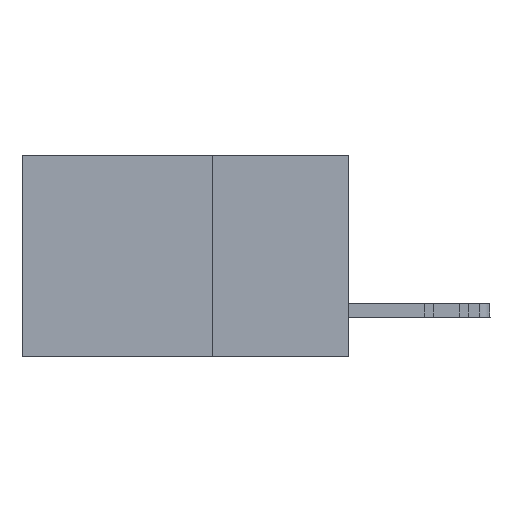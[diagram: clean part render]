
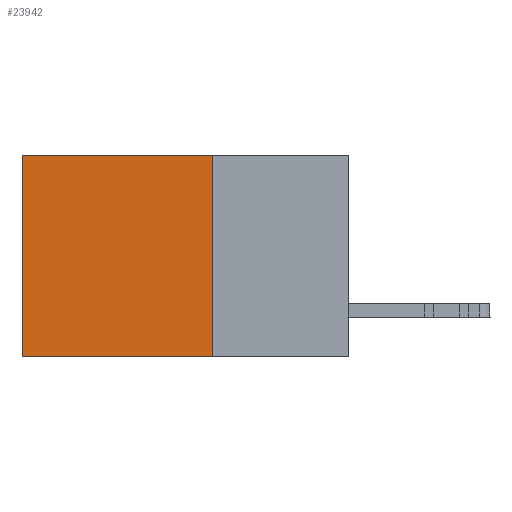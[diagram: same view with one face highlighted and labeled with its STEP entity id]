
A CAD part, left-side view. The second image highlights one B-rep face of the part: STEP entity #23942.
In plain terms, the highlighted planar face has unit normal (-1, 0, 0).
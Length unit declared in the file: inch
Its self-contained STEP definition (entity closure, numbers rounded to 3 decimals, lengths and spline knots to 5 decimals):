
#13 = DIRECTION ( 'NONE',  ( 1., 0., 0. ) ) ;
#1052 = EDGE_CURVE ( 'NONE', #3298, #9524, #8488, .T. ) ;
#1216 = VERTEX_POINT ( 'NONE', #14364 ) ;
#2584 = DIRECTION ( 'NONE',  ( 0., 0., -1. ) ) ;
#2949 = EDGE_CURVE ( 'NONE', #5682, #3298, #21023, .T. ) ;
#3145 = CARTESIAN_POINT ( 'NONE',  ( 0.298, 0.25, -0.37 ) ) ;
#3233 = VECTOR ( 'NONE', #11084, 39.37008 ) ;
#3298 = VERTEX_POINT ( 'NONE', #3145 ) ;
#4064 = DIRECTION ( 'NONE',  ( 0., 0., -1. ) ) ;
#4912 = FACE_OUTER_BOUND ( 'NONE', #11764, .T. ) ;
#4947 = VECTOR ( 'NONE', #11719, 39.37008 ) ;
#5124 = CARTESIAN_POINT ( 'NONE',  ( 0.298, 0.25, 0. ) ) ;
#5374 = CARTESIAN_POINT ( 'NONE',  ( 0.298, 0.6, -0.37 ) ) ;
#5555 = CARTESIAN_POINT ( 'NONE',  ( 0.298, 0.6, 0. ) ) ;
#5682 = VERTEX_POINT ( 'NONE', #8349 ) ;
#5852 = ORIENTED_EDGE ( 'NONE', *, *, #26407, .T. ) ;
#6251 = CARTESIAN_POINT ( 'NONE',  ( 0.298, 0.25, 0. ) ) ;
#6749 = VECTOR ( 'NONE', #2584, 39.37008 ) ;
#7131 = LINE ( 'NONE', #5124, #3233 ) ;
#7224 = EDGE_CURVE ( 'NONE', #5682, #1216, #7131, .T. ) ;
#8349 = CARTESIAN_POINT ( 'NONE',  ( 0.298, 0.25, 0. ) ) ;
#8488 = LINE ( 'NONE', #19992, #4947 ) ;
#8994 = LINE ( 'NONE', #5555, #22265 ) ;
#9524 = VERTEX_POINT ( 'NONE', #5374 ) ;
#9653 = ORIENTED_EDGE ( 'NONE', *, *, #1052, .F. ) ;
#11084 = DIRECTION ( 'NONE',  ( 0., 1., 0. ) ) ;
#11719 = DIRECTION ( 'NONE',  ( 0., 1., 0. ) ) ;
#11764 = EDGE_LOOP ( 'NONE', ( #5852, #9653, #14864, #23174 ) ) ;
#14364 = CARTESIAN_POINT ( 'NONE',  ( 0.298, 0.6, 0. ) ) ;
#14864 = ORIENTED_EDGE ( 'NONE', *, *, #2949, .F. ) ;
#19992 = CARTESIAN_POINT ( 'NONE',  ( 0.298, 0.25, -0.37 ) ) ;
#20626 = PLANE ( 'NONE',  #20905 ) ;
#20905 = AXIS2_PLACEMENT_3D ( 'NONE', #6251, #13, #4064 ) ;
#21023 = LINE ( 'NONE', #23589, #6749 ) ;
#22265 = VECTOR ( 'NONE', #24212, 39.37008 ) ;
#23174 = ORIENTED_EDGE ( 'NONE', *, *, #7224, .T. ) ;
#23589 = CARTESIAN_POINT ( 'NONE',  ( 0.298, 0.25, 0. ) ) ;
#23942 = ADVANCED_FACE ( 'NONE', ( #4912 ), #20626, .F. ) ;
#24212 = DIRECTION ( 'NONE',  ( 0., 0., -1. ) ) ;
#26407 = EDGE_CURVE ( 'NONE', #1216, #9524, #8994, .T. ) ;
